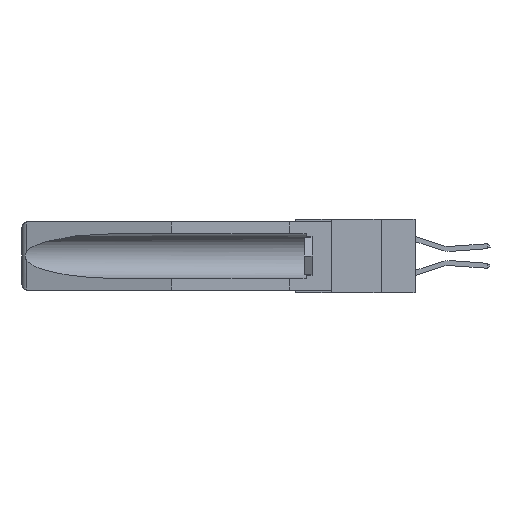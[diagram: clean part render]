
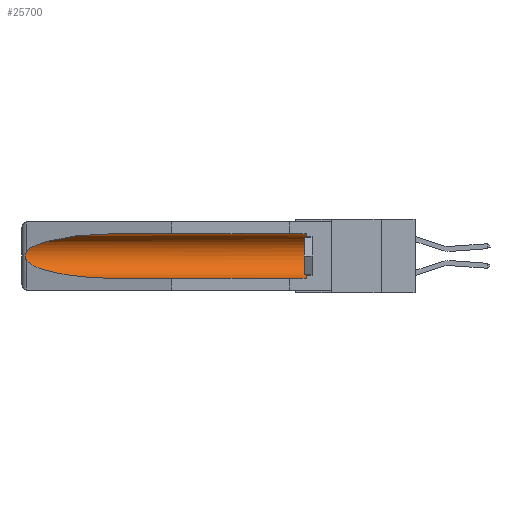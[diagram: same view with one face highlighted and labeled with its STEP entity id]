
A CAD part, left-side view. The second image highlights one B-rep face of the part: STEP entity #25700.
In plain terms, the highlighted cylindrical face has radius 2.857 mm (diameter 5.715 mm), a partial arc.
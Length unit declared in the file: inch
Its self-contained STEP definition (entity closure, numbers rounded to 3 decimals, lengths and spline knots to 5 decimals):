
#990 = EDGE_CURVE ( 'NONE', #7172, #4055, #25453, .T. ) ;
#1323 = EDGE_CURVE ( 'NONE', #25513, #30776, #9149, .T. ) ;
#1841 = VECTOR ( 'NONE', #6925, 39.37008 ) ;
#1943 = CARTESIAN_POINT ( 'NONE',  ( 0.26537, 1.52718, -0.19328 ) ) ;
#2020 = CARTESIAN_POINT ( 'NONE',  ( 0.26597, 1.5296, -0.19026 ) ) ;
#3309 = CARTESIAN_POINT ( 'NONE',  ( 0.2673, 1.5327, -0.16383 ) ) ;
#3830 = ORIENTED_EDGE ( 'NONE', *, *, #990, .T. ) ;
#3847 = EDGE_CURVE ( 'NONE', #14415, #25513, #23994, .T. ) ;
#4055 = VERTEX_POINT ( 'NONE', #13700 ) ;
#4354 = AXIS2_PLACEMENT_3D ( 'NONE', #4597, #19215, #9373 ) ;
#4597 = CARTESIAN_POINT ( 'NONE',  ( 0.155, 0.126, -0.1715 ) ) ;
#5405 = ORIENTED_EDGE ( 'NONE', *, *, #1323, .T. ) ;
#5797 = VERTEX_POINT ( 'NONE', #28011 ) ;
#5952 = CARTESIAN_POINT ( 'NONE',  ( 0.21114, 1.30732, -0.059 ) ) ;
#6262 = CARTESIAN_POINT ( 'NONE',  ( 0.26654, 1.53092, -0.15636 ) ) ;
#6518 = CARTESIAN_POINT ( 'NONE',  ( 0.26597, 1.52961, -0.15275 ) ) ;
#6925 = DIRECTION ( 'NONE',  ( 0., 1., 0. ) ) ;
#7084 = DIRECTION ( 'NONE',  ( 0., 1., 0. ) ) ;
#7172 = VERTEX_POINT ( 'NONE', #17460 ) ;
#7801 = CARTESIAN_POINT ( 'NONE',  ( 0.155, 1.07973, -0.059 ) ) ;
#8683 = CARTESIAN_POINT ( 'NONE',  ( 0.26655, 1.53094, -0.18657 ) ) ;
#9149 =( BOUNDED_CURVE ( )  B_SPLINE_CURVE ( 3, ( #32006, #31897, #21755, #19486 ),
 .UNSPECIFIED., .F., .F. ) 
 B_SPLINE_CURVE_WITH_KNOTS ( ( 4, 4 ),
 ( 0.1948, 1.5708 ),
 .UNSPECIFIED. ) 
 CURVE ( )  GEOMETRIC_REPRESENTATION_ITEM ( )  RATIONAL_B_SPLINE_CURVE ( ( 1., 0.848, 0.848, 1. ) ) 
 REPRESENTATION_ITEM ( '' )  );
#9250 = CARTESIAN_POINT ( 'NONE',  ( 0.155, -0.30754, -0.059 ) ) ;
#9373 = DIRECTION ( 'NONE',  ( 0., 0., 1. ) ) ;
#9547 =( BOUNDED_CURVE ( )  B_SPLINE_CURVE ( 3, ( #7801, #5952, #13450, #30696 ),
 .UNSPECIFIED., .F., .F. ) 
 B_SPLINE_CURVE_WITH_KNOTS ( ( 4, 4 ),
 ( 4.71239, 6.08839 ),
 .UNSPECIFIED. ) 
 CURVE ( )  GEOMETRIC_REPRESENTATION_ITEM ( )  RATIONAL_B_SPLINE_CURVE ( ( 1., 0.848, 0.848, 1. ) ) 
 REPRESENTATION_ITEM ( '' )  );
#11792 = CARTESIAN_POINT ( 'NONE',  ( 0.2675, 1.53308, -0.17534 ) ) ;
#13450 = CARTESIAN_POINT ( 'NONE',  ( 0.25451, 1.48313, -0.09465 ) ) ;
#13700 = CARTESIAN_POINT ( 'NONE',  ( 0.155, 0.126, -0.059 ) ) ;
#14044 = DIRECTION ( 'NONE',  ( 0., 1., 0. ) ) ;
#14415 = VERTEX_POINT ( 'NONE', #23672 ) ;
#14835 = CYLINDRICAL_SURFACE ( 'NONE', #18132, 0.1125 ) ;
#17460 = CARTESIAN_POINT ( 'NONE',  ( 0.155, 0.126, -0.284 ) ) ;
#17596 = ORIENTED_EDGE ( 'NONE', *, *, #28244, .T. ) ;
#18132 = AXIS2_PLACEMENT_3D ( 'NONE', #29201, #7084, #27127 ) ;
#19215 = DIRECTION ( 'NONE',  ( 0., -1., 0. ) ) ;
#19486 = CARTESIAN_POINT ( 'NONE',  ( 0.155, 1.07973, -0.284 ) ) ;
#19890 = EDGE_CURVE ( 'NONE', #7172, #30776, #23894, .T. ) ;
#20483 = ORIENTED_EDGE ( 'NONE', *, *, #19890, .F. ) ;
#21341 = CARTESIAN_POINT ( 'NONE',  ( 0.155, 1.07973, -0.284 ) ) ;
#21591 = LINE ( 'NONE', #9250, #27362 ) ;
#21755 = CARTESIAN_POINT ( 'NONE',  ( 0.21114, 1.30732, -0.284 ) ) ;
#21804 = CARTESIAN_POINT ( 'NONE',  ( 0.26537, 1.52718, -0.19328 ) ) ;
#23672 = CARTESIAN_POINT ( 'NONE',  ( 0.26537, 1.52718, -0.14972 ) ) ;
#23894 = LINE ( 'NONE', #26556, #1841 ) ;
#23994 = B_SPLINE_CURVE_WITH_KNOTS ( 'NONE', 3,
 ( #27790, #6518, #6262, #3309, #30970, #11792, #24117, #8683, #2020, #21804 ),
 .UNSPECIFIED., .F., .F.,
 ( 4, 2, 2, 2, 4 ),
 ( 0., 0.00029, 0.00058, 0.00087, 0.00117 ),
 .UNSPECIFIED. ) ;
#24117 = CARTESIAN_POINT ( 'NONE',  ( 0.2673, 1.53269, -0.17917 ) ) ;
#24131 = ORIENTED_EDGE ( 'NONE', *, *, #26631, .T. ) ;
#25453 = CIRCLE ( 'NONE', #4354, 0.1125 ) ;
#25513 = VERTEX_POINT ( 'NONE', #1943 ) ;
#25700 = ADVANCED_FACE ( 'NONE', ( #29072 ), #14835, .F. ) ;
#26556 = CARTESIAN_POINT ( 'NONE',  ( 0.155, -0.30754, -0.284 ) ) ;
#26631 = EDGE_CURVE ( 'NONE', #5797, #14415, #9547, .T. ) ;
#27127 = DIRECTION ( 'NONE',  ( 0., 0., 1. ) ) ;
#27362 = VECTOR ( 'NONE', #14044, 39.37008 ) ;
#27671 = EDGE_LOOP ( 'NONE', ( #24131, #30973, #5405, #20483, #3830, #17596 ) ) ;
#27790 = CARTESIAN_POINT ( 'NONE',  ( 0.26537, 1.52718, -0.14972 ) ) ;
#28011 = CARTESIAN_POINT ( 'NONE',  ( 0.155, 1.07973, -0.059 ) ) ;
#28244 = EDGE_CURVE ( 'NONE', #4055, #5797, #21591, .T. ) ;
#29072 = FACE_OUTER_BOUND ( 'NONE', #27671, .T. ) ;
#29201 = CARTESIAN_POINT ( 'NONE',  ( 0.155, -0.30754, -0.1715 ) ) ;
#30696 = CARTESIAN_POINT ( 'NONE',  ( 0.26537, 1.52718, -0.14972 ) ) ;
#30776 = VERTEX_POINT ( 'NONE', #21341 ) ;
#30970 = CARTESIAN_POINT ( 'NONE',  ( 0.2675, 1.53308, -0.16763 ) ) ;
#30973 = ORIENTED_EDGE ( 'NONE', *, *, #3847, .T. ) ;
#31897 = CARTESIAN_POINT ( 'NONE',  ( 0.25451, 1.48313, -0.24835 ) ) ;
#32006 = CARTESIAN_POINT ( 'NONE',  ( 0.26537, 1.52718, -0.19328 ) ) ;
